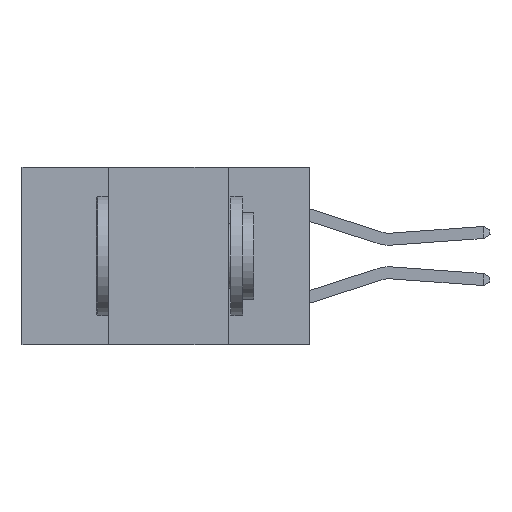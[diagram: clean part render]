
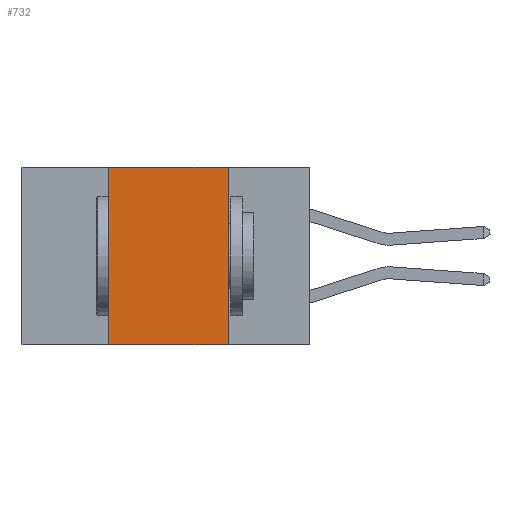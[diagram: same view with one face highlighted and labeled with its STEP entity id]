
A CAD part, left-side view. The second image highlights one B-rep face of the part: STEP entity #732.
In plain terms, the highlighted planar face has unit normal (-1, 0, 0).
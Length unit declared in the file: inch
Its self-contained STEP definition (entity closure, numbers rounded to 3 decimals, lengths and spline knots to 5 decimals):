
#589 = LINE ( 'NONE', #7444, #1755 ) ;
#732 = ADVANCED_FACE ( 'NONE', ( #2577 ), #12741, .F. ) ;
#1056 = CARTESIAN_POINT ( 'NONE',  ( 0., 0.17, -0.37 ) ) ;
#1497 = VECTOR ( 'NONE', #4318, 39.37008 ) ;
#1755 = VECTOR ( 'NONE', #10463, 39.37008 ) ;
#1835 = DIRECTION ( 'NONE',  ( 0., 0., 1. ) ) ;
#2104 = CARTESIAN_POINT ( 'NONE',  ( 0., 0.42, 0. ) ) ;
#2114 = AXIS2_PLACEMENT_3D ( 'NONE', #13790, #13712, #11641 ) ;
#2577 = FACE_OUTER_BOUND ( 'NONE', #8339, .T. ) ;
#2791 = LINE ( 'NONE', #11926, #12783 ) ;
#3155 = ORIENTED_EDGE ( 'NONE', *, *, #13123, .F. ) ;
#3337 = LINE ( 'NONE', #1056, #1497 ) ;
#4144 = CARTESIAN_POINT ( 'NONE',  ( 0., 0.6, -0.37 ) ) ;
#4318 = DIRECTION ( 'NONE',  ( 0., 0., -1. ) ) ;
#4382 = VERTEX_POINT ( 'NONE', #2104 ) ;
#4951 = DIRECTION ( 'NONE',  ( 0., -1., 0. ) ) ;
#5545 = CARTESIAN_POINT ( 'NONE',  ( 0., 0.17, -0.37 ) ) ;
#5840 = ORIENTED_EDGE ( 'NONE', *, *, #7085, .F. ) ;
#6439 = VECTOR ( 'NONE', #4951, 39.37008 ) ;
#6516 = EDGE_CURVE ( 'NONE', #13656, #4382, #2791, .T. ) ;
#7085 = EDGE_CURVE ( 'NONE', #11802, #8984, #3337, .T. ) ;
#7444 = CARTESIAN_POINT ( 'NONE',  ( 0., 0.6, 0. ) ) ;
#8339 = EDGE_LOOP ( 'NONE', ( #5840, #3155, #11616, #10157 ) ) ;
#8583 = LINE ( 'NONE', #4144, #6439 ) ;
#8898 = CARTESIAN_POINT ( 'NONE',  ( 0., 0.42, -0.37 ) ) ;
#8984 = VERTEX_POINT ( 'NONE', #5545 ) ;
#10157 = ORIENTED_EDGE ( 'NONE', *, *, #12454, .T. ) ;
#10463 = DIRECTION ( 'NONE',  ( 0., -1., 0. ) ) ;
#11616 = ORIENTED_EDGE ( 'NONE', *, *, #6516, .F. ) ;
#11641 = DIRECTION ( 'NONE',  ( 0., 0., -1. ) ) ;
#11802 = VERTEX_POINT ( 'NONE', #11930 ) ;
#11926 = CARTESIAN_POINT ( 'NONE',  ( 0., 0.42, -0.37 ) ) ;
#11930 = CARTESIAN_POINT ( 'NONE',  ( 0., 0.17, 0. ) ) ;
#12454 = EDGE_CURVE ( 'NONE', #13656, #8984, #8583, .T. ) ;
#12741 = PLANE ( 'NONE',  #2114 ) ;
#12783 = VECTOR ( 'NONE', #1835, 39.37008 ) ;
#13123 = EDGE_CURVE ( 'NONE', #4382, #11802, #589, .T. ) ;
#13656 = VERTEX_POINT ( 'NONE', #8898 ) ;
#13712 = DIRECTION ( 'NONE',  ( 1., 0., 0. ) ) ;
#13790 = CARTESIAN_POINT ( 'NONE',  ( 0., 0.6, 0. ) ) ;
